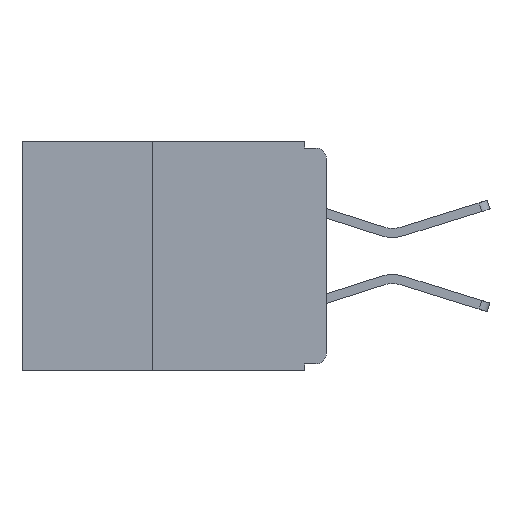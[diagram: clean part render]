
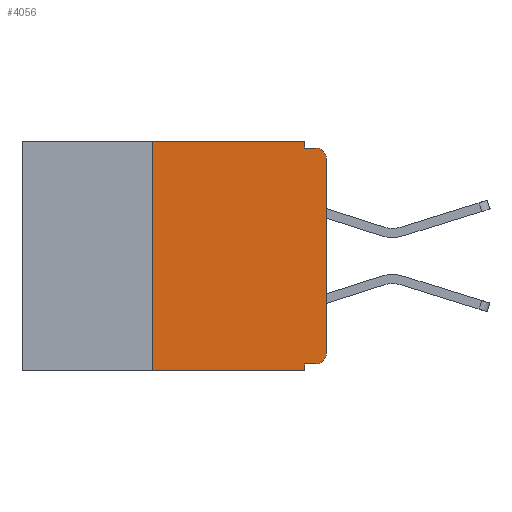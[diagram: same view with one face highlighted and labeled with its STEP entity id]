
A CAD part, left-side view. The second image highlights one B-rep face of the part: STEP entity #4056.
In plain terms, the highlighted planar face has unit normal (-1, 0, 0).
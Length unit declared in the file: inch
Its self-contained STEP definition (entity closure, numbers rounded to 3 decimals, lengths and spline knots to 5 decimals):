
#324 = VERTEX_POINT ( 'NONE', #23977 ) ;
#465 = EDGE_CURVE ( 'NONE', #24944, #25128, #22444, .T. ) ;
#541 = VECTOR ( 'NONE', #13279, 39.37008 ) ;
#557 = ORIENTED_EDGE ( 'NONE', *, *, #3521, .T. ) ;
#577 = DIRECTION ( 'NONE',  ( 0., -1., 0. ) ) ;
#1035 = EDGE_CURVE ( 'NONE', #8330, #1326, #24824, .T. ) ;
#1111 = CIRCLE ( 'NONE', #22186, 0.015 ) ;
#1326 = VERTEX_POINT ( 'NONE', #6786 ) ;
#2100 = ORIENTED_EDGE ( 'NONE', *, *, #19224, .T. ) ;
#2159 = EDGE_CURVE ( 'NONE', #8330, #18852, #19325, .T. ) ;
#2305 = AXIS2_PLACEMENT_3D ( 'NONE', #11829, #11514, #11489 ) ;
#2382 = EDGE_CURVE ( 'NONE', #1326, #16962, #24147, .T. ) ;
#2417 = ORIENTED_EDGE ( 'NONE', *, *, #1035, .F. ) ;
#2595 = DIRECTION ( 'NONE',  ( 0., -1., 0. ) ) ;
#2597 = AXIS2_PLACEMENT_3D ( 'NONE', #24567, #24427, #24293 ) ;
#3024 = LINE ( 'NONE', #14301, #13447 ) ;
#3521 = EDGE_CURVE ( 'NONE', #7387, #16962, #7732, .T. ) ;
#3962 = ORIENTED_EDGE ( 'NONE', *, *, #5428, .F. ) ;
#4056 = ADVANCED_FACE ( 'NONE', ( #17482 ), #11892, .F. ) ;
#5428 = EDGE_CURVE ( 'NONE', #25128, #324, #5781, .T. ) ;
#5601 = CARTESIAN_POINT ( 'NONE',  ( 0., 0., 0. ) ) ;
#5781 = LINE ( 'NONE', #13365, #541 ) ;
#6039 = CARTESIAN_POINT ( 'NONE',  ( 0., 0.25, -0.33 ) ) ;
#6202 = CARTESIAN_POINT ( 'NONE',  ( 0., 0.25, -0.33 ) ) ;
#6786 = CARTESIAN_POINT ( 'NONE',  ( 0., 0.031, -0.32 ) ) ;
#7189 = CARTESIAN_POINT ( 'NONE',  ( 0., 0., -0.32 ) ) ;
#7387 = VERTEX_POINT ( 'NONE', #6202 ) ;
#7404 = LINE ( 'NONE', #5601, #22230 ) ;
#7428 = DIRECTION ( 'NONE',  ( -1., 0., 0. ) ) ;
#7732 = LINE ( 'NONE', #18099, #22559 ) ;
#8011 = DIRECTION ( 'NONE',  ( 0., 0., 1. ) ) ;
#8257 = DIRECTION ( 'NONE',  ( 0., 1., 0. ) ) ;
#8330 = VERTEX_POINT ( 'NONE', #9183 ) ;
#9155 = ORIENTED_EDGE ( 'NONE', *, *, #465, .F. ) ;
#9183 = CARTESIAN_POINT ( 'NONE',  ( 0., 0.015, -0.32 ) ) ;
#9309 = LINE ( 'NONE', #6039, #18998 ) ;
#9548 = CARTESIAN_POINT ( 'NONE',  ( 0., 0., -0.025 ) ) ;
#10013 = VECTOR ( 'NONE', #8257, 39.37008 ) ;
#11086 = EDGE_CURVE ( 'NONE', #18852, #16549, #7404, .T. ) ;
#11489 = DIRECTION ( 'NONE',  ( 0., 0., -1. ) ) ;
#11514 = DIRECTION ( 'NONE',  ( 1., 0., 0. ) ) ;
#11621 = ORIENTED_EDGE ( 'NONE', *, *, #2382, .F. ) ;
#11829 = CARTESIAN_POINT ( 'NONE',  ( 0., 0.437, 0. ) ) ;
#11892 = PLANE ( 'NONE',  #2305 ) ;
#12136 = CARTESIAN_POINT ( 'NONE',  ( 0., 0., -0.305 ) ) ;
#12188 = VECTOR ( 'NONE', #2595, 39.37008 ) ;
#13279 = DIRECTION ( 'NONE',  ( 0., 0., -1. ) ) ;
#13365 = CARTESIAN_POINT ( 'NONE',  ( 0., 0.031, 0. ) ) ;
#13447 = VECTOR ( 'NONE', #577, 39.37008 ) ;
#13630 = VERTEX_POINT ( 'NONE', #17563 ) ;
#14016 = CARTESIAN_POINT ( 'NONE',  ( 0., 0.25, 0. ) ) ;
#14301 = CARTESIAN_POINT ( 'NONE',  ( 0., 0., -0.01 ) ) ;
#14772 = EDGE_CURVE ( 'NONE', #7387, #24944, #9309, .T. ) ;
#15552 = ORIENTED_EDGE ( 'NONE', *, *, #14772, .F. ) ;
#15681 = CARTESIAN_POINT ( 'NONE',  ( 0., 0.031, -0.33 ) ) ;
#15839 = ORIENTED_EDGE ( 'NONE', *, *, #11086, .T. ) ;
#16418 = CARTESIAN_POINT ( 'NONE',  ( 0., 0.031, 0. ) ) ;
#16549 = VERTEX_POINT ( 'NONE', #9548 ) ;
#16939 = DIRECTION ( 'NONE',  ( 0., 0., -1. ) ) ;
#16962 = VERTEX_POINT ( 'NONE', #15681 ) ;
#17370 = CARTESIAN_POINT ( 'NONE',  ( 0., 0.031, -0.33 ) ) ;
#17482 = FACE_OUTER_BOUND ( 'NONE', #18277, .T. ) ;
#17563 = CARTESIAN_POINT ( 'NONE',  ( 0., 0.015, -0.01 ) ) ;
#18072 = DIRECTION ( 'NONE',  ( 0., -1., 0. ) ) ;
#18099 = CARTESIAN_POINT ( 'NONE',  ( 0., 0.437, -0.33 ) ) ;
#18251 = EDGE_CURVE ( 'NONE', #324, #13630, #3024, .T. ) ;
#18277 = EDGE_LOOP ( 'NONE', ( #15839, #2100, #22785, #3962, #9155, #15552, #557, #11621, #2417, #23702 ) ) ;
#18392 = VECTOR ( 'NONE', #16939, 39.37008 ) ;
#18852 = VERTEX_POINT ( 'NONE', #12136 ) ;
#18998 = VECTOR ( 'NONE', #8011, 39.37008 ) ;
#19017 = CARTESIAN_POINT ( 'NONE',  ( 0., 0.015, -0.025 ) ) ;
#19224 = EDGE_CURVE ( 'NONE', #16549, #13630, #1111, .T. ) ;
#19325 = CIRCLE ( 'NONE', #2597, 0.015 ) ;
#20961 = DIRECTION ( 'NONE',  ( 0., 0., -1. ) ) ;
#22186 = AXIS2_PLACEMENT_3D ( 'NONE', #19017, #7428, #20961 ) ;
#22212 = CARTESIAN_POINT ( 'NONE',  ( 0., 0.437, 0. ) ) ;
#22230 = VECTOR ( 'NONE', #23002, 39.37008 ) ;
#22444 = LINE ( 'NONE', #22212, #12188 ) ;
#22559 = VECTOR ( 'NONE', #18072, 39.37008 ) ;
#22785 = ORIENTED_EDGE ( 'NONE', *, *, #18251, .F. ) ;
#23002 = DIRECTION ( 'NONE',  ( 0., 0., 1. ) ) ;
#23702 = ORIENTED_EDGE ( 'NONE', *, *, #2159, .T. ) ;
#23977 = CARTESIAN_POINT ( 'NONE',  ( 0., 0.031, -0.01 ) ) ;
#24147 = LINE ( 'NONE', #17370, #18392 ) ;
#24293 = DIRECTION ( 'NONE',  ( 0., 0., -1. ) ) ;
#24427 = DIRECTION ( 'NONE',  ( -1., 0., 0. ) ) ;
#24567 = CARTESIAN_POINT ( 'NONE',  ( 0., 0.015, -0.305 ) ) ;
#24824 = LINE ( 'NONE', #7189, #10013 ) ;
#24944 = VERTEX_POINT ( 'NONE', #14016 ) ;
#25128 = VERTEX_POINT ( 'NONE', #16418 ) ;
